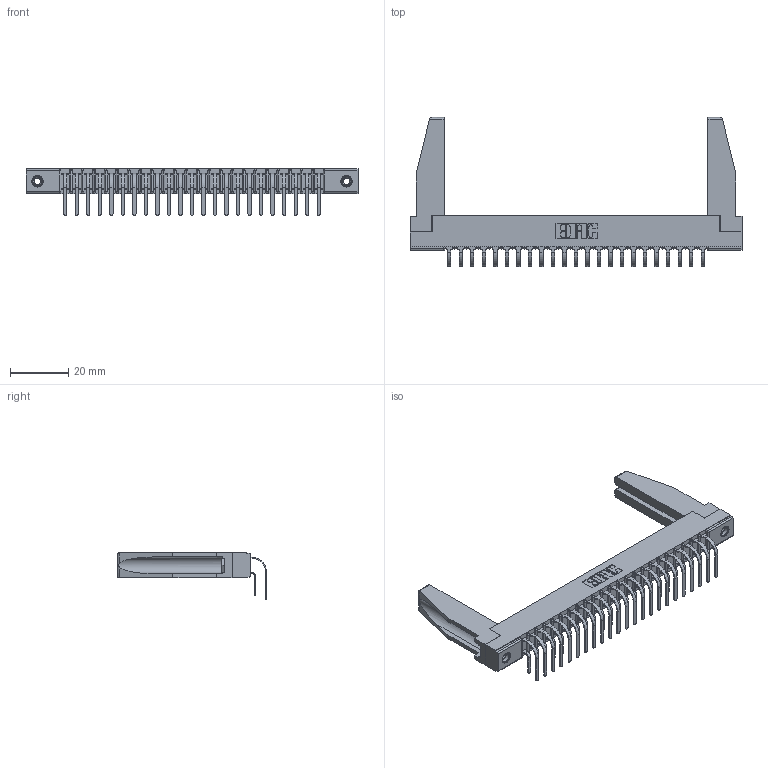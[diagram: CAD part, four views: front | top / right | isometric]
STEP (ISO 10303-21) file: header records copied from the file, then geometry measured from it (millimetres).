
FILE_DESCRIPTION (( 'STEP AP203' ), '1' );
FILE_NAME ('357-046-459-278.STEP', '2022-07-07T23:06:32', ( '' ), ( '' ), 'SwSTEP 2.0', 'SolidWorks 2020', '' );
FILE_SCHEMA (( 'CONFIG_CONTROL_DESIGN' ));
Length unit declared in the file: inch
Products named in the file (6): 307-290-001_559 - 2 (Single); 307-220-078; 307 Part_.156 Dia Mounting Holes; 357-046-459-278; 345-250-001_345-250-001-102; 307-290-001_558 559 - 1 (Single)
Assembly tree (51 placements, depth 2):
  357-046-459-278
    307 Part_.156 Dia Mounting Holes
    307-290-001_558 559 - 1 (Single)  x23
    307-290-001_559 - 2 (Single)  x23
    307-220-078  x2
    345-250-001_345-250-001-102  x2
Bounding box: 114.15 x 51.22 x 16.08 mm (x, y, z)
Volume: 11632.7 mm3; surface area: 18331.6 mm2
Topology: 51 solids, 51 shells, 2572 faces, 7185 edges, 4654 vertices
Faces by surface type: plane 1672, cylinder 836, sphere 48, cone 12, torus 4
Entity records: 26682 total; most frequent: CARTESIAN_POINT 4383, ORIENTED_EDGE 4300, DIRECTION 4254, EDGE_CURVE 2150, VECTOR 1644, LINE 1644, VERTEX_POINT 1392, AXIS2_PLACEMENT_3D 1305
